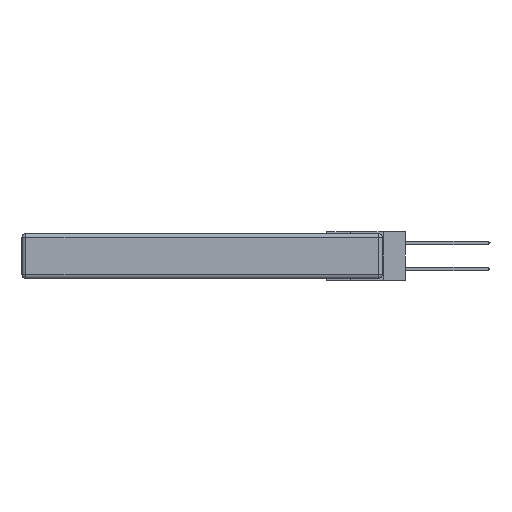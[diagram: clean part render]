
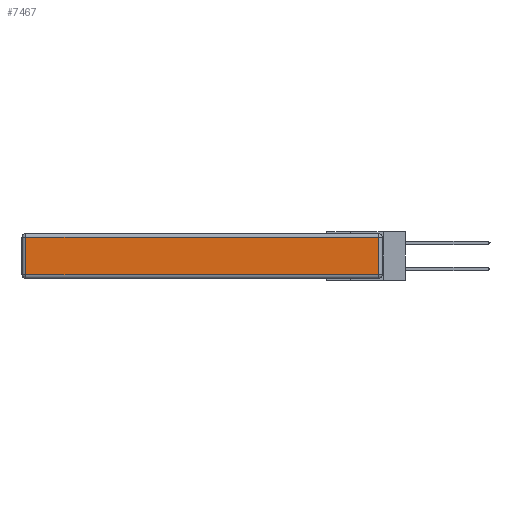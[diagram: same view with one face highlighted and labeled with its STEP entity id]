
A CAD part, left-side view. The second image highlights one B-rep face of the part: STEP entity #7467.
In plain terms, the highlighted planar face has unit normal (-1, 0, 0).
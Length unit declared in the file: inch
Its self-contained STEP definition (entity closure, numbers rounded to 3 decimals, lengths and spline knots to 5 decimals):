
#940 = EDGE_CURVE ( 'NONE', #8629, #28526, #21564, .T. ) ;
#1372 = DIRECTION ( 'NONE',  ( 0., 0., 1. ) ) ;
#1911 = DIRECTION ( 'NONE',  ( 0., 0., -1. ) ) ;
#2040 = CARTESIAN_POINT ( 'NONE',  ( 0., 2.75, -0.03 ) ) ;
#2578 = VERTEX_POINT ( 'NONE', #25392 ) ;
#2821 = PLANE ( 'NONE',  #13608 ) ;
#3756 = EDGE_CURVE ( 'NONE', #28526, #2578, #5262, .T. ) ;
#4349 = ORIENTED_EDGE ( 'NONE', *, *, #3756, .T. ) ;
#4873 = VECTOR ( 'NONE', #1372, 39.37008 ) ;
#4935 = CARTESIAN_POINT ( 'NONE',  ( 0., 2.72, -0.313 ) ) ;
#5262 = LINE ( 'NONE', #14815, #29468 ) ;
#6333 = LINE ( 'NONE', #19813, #4873 ) ;
#6387 = ORIENTED_EDGE ( 'NONE', *, *, #27094, .T. ) ;
#6845 = ORIENTED_EDGE ( 'NONE', *, *, #940, .T. ) ;
#6884 = DIRECTION ( 'NONE',  ( 0., 1., 0. ) ) ;
#7467 = ADVANCED_FACE ( 'NONE', ( #19782 ), #2821, .T. ) ;
#8629 = VERTEX_POINT ( 'NONE', #26442 ) ;
#9097 = CARTESIAN_POINT ( 'NONE',  ( 0., 0.03, -0.03 ) ) ;
#9331 = CARTESIAN_POINT ( 'NONE',  ( 0., 0., -0.343 ) ) ;
#9515 = EDGE_LOOP ( 'NONE', ( #4349, #16047, #6387, #6845 ) ) ;
#10853 = EDGE_CURVE ( 'NONE', #2578, #22697, #6333, .T. ) ;
#13608 = AXIS2_PLACEMENT_3D ( 'NONE', #9331, #23595, #28462 ) ;
#14762 = LINE ( 'NONE', #2040, #27906 ) ;
#14815 = CARTESIAN_POINT ( 'NONE',  ( 0., 0., -0.313 ) ) ;
#16047 = ORIENTED_EDGE ( 'NONE', *, *, #10853, .T. ) ;
#19782 = FACE_OUTER_BOUND ( 'NONE', #9515, .T. ) ;
#19813 = CARTESIAN_POINT ( 'NONE',  ( 0., 0.03, -0.343 ) ) ;
#21564 = LINE ( 'NONE', #25339, #24520 ) ;
#22697 = VERTEX_POINT ( 'NONE', #9097 ) ;
#23595 = DIRECTION ( 'NONE',  ( -1., 0., 0. ) ) ;
#24520 = VECTOR ( 'NONE', #1911, 39.37008 ) ;
#25339 = CARTESIAN_POINT ( 'NONE',  ( 0., 2.72, -0.343 ) ) ;
#25392 = CARTESIAN_POINT ( 'NONE',  ( 0., 0.03, -0.313 ) ) ;
#26373 = DIRECTION ( 'NONE',  ( 0., -1., 0. ) ) ;
#26442 = CARTESIAN_POINT ( 'NONE',  ( 0., 2.72, -0.03 ) ) ;
#27094 = EDGE_CURVE ( 'NONE', #22697, #8629, #14762, .T. ) ;
#27906 = VECTOR ( 'NONE', #6884, 39.37008 ) ;
#28462 = DIRECTION ( 'NONE',  ( 0., 0., 1. ) ) ;
#28526 = VERTEX_POINT ( 'NONE', #4935 ) ;
#29468 = VECTOR ( 'NONE', #26373, 39.37008 ) ;
